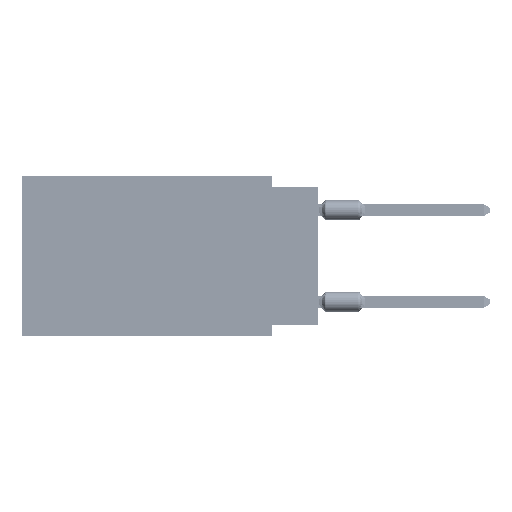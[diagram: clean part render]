
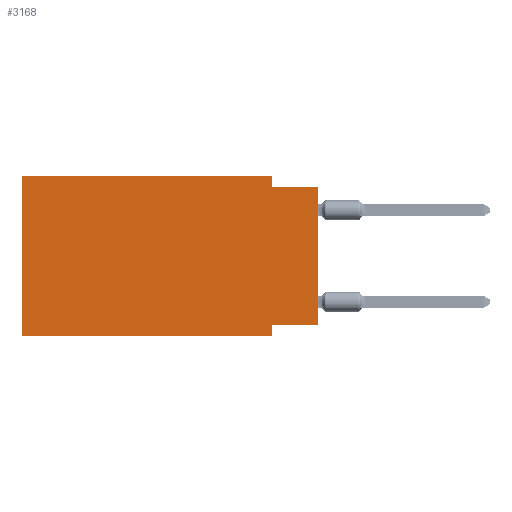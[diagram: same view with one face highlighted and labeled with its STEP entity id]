
A CAD part, left-side view. The second image highlights one B-rep face of the part: STEP entity #3168.
In plain terms, the highlighted planar face has unit normal (-1, 0, 0).
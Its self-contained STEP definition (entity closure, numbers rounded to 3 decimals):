
#1804 = VECTOR ( 'NONE', #104133, 1000. ) ;
#2034 = EDGE_CURVE ( 'NONE', #8779, #92417, #47428, .T. ) ;
#2912 = CARTESIAN_POINT ( 'NONE',  ( 0., 16.383, -8.89 ) ) ;
#3168 = ADVANCED_FACE ( 'NONE', ( #45358 ), #28938, .F. ) ;
#7784 = ORIENTED_EDGE ( 'NONE', *, *, #20127, .T. ) ;
#8779 = VERTEX_POINT ( 'NONE', #37899 ) ;
#11572 = ORIENTED_EDGE ( 'NONE', *, *, #51836, .F. ) ;
#13148 = ORIENTED_EDGE ( 'NONE', *, *, #77947, .F. ) ;
#14247 = DIRECTION ( 'NONE',  ( 0., -1., 0. ) ) ;
#14789 = VECTOR ( 'NONE', #48491, 1000. ) ;
#17339 = VERTEX_POINT ( 'NONE', #75725 ) ;
#20127 = EDGE_CURVE ( 'NONE', #87965, #74769, #34711, .T. ) ;
#21011 = DIRECTION ( 'NONE',  ( 1., 0., 0. ) ) ;
#26258 = EDGE_CURVE ( 'NONE', #67999, #33209, #50762, .T. ) ;
#26280 = CARTESIAN_POINT ( 'NONE',  ( 0., 16.383, -8.89 ) ) ;
#26295 = VECTOR ( 'NONE', #99499, 1000. ) ;
#27564 = CARTESIAN_POINT ( 'NONE',  ( 0., 2.54, -8.255 ) ) ;
#28281 = EDGE_CURVE ( 'NONE', #92417, #17339, #39917, .T. ) ;
#28938 = PLANE ( 'NONE',  #81557 ) ;
#29071 = CARTESIAN_POINT ( 'NONE',  ( 0., 16.383, 0. ) ) ;
#33209 = VERTEX_POINT ( 'NONE', #27564 ) ;
#34711 = LINE ( 'NONE', #2912, #74892 ) ;
#36169 = EDGE_LOOP ( 'NONE', ( #53392, #39734, #96352, #13148, #97157, #7784, #11572, #40665 ) ) ;
#37899 = CARTESIAN_POINT ( 'NONE',  ( 0., 2.54, 0. ) ) ;
#39734 = ORIENTED_EDGE ( 'NONE', *, *, #28281, .F. ) ;
#39737 = CARTESIAN_POINT ( 'NONE',  ( 0., 2.54, -0.635 ) ) ;
#39917 = LINE ( 'NONE', #71740, #100987 ) ;
#40665 = ORIENTED_EDGE ( 'NONE', *, *, #26258, .F. ) ;
#41595 = LINE ( 'NONE', #56988, #103772 ) ;
#45358 = FACE_OUTER_BOUND ( 'NONE', #36169, .T. ) ;
#47428 = LINE ( 'NONE', #82246, #1804 ) ;
#48491 = DIRECTION ( 'NONE',  ( 0., 0., 1. ) ) ;
#49646 = CARTESIAN_POINT ( 'NONE',  ( 0., 0., -8.255 ) ) ;
#50762 = LINE ( 'NONE', #83106, #26295 ) ;
#51836 = EDGE_CURVE ( 'NONE', #33209, #74769, #41595, .T. ) ;
#52178 = LINE ( 'NONE', #94553, #97591 ) ;
#53312 = DIRECTION ( 'NONE',  ( 0., 0., -1. ) ) ;
#53392 = ORIENTED_EDGE ( 'NONE', *, *, #82528, .T. ) ;
#54285 = DIRECTION ( 'NONE',  ( 0., 0., 1. ) ) ;
#56531 = EDGE_CURVE ( 'NONE', #87965, #81374, #64407, .T. ) ;
#56988 = CARTESIAN_POINT ( 'NONE',  ( 0., 2.54, -8.89 ) ) ;
#64407 = LINE ( 'NONE', #72886, #14789 ) ;
#67553 = DIRECTION ( 'NONE',  ( 0., -1., 0. ) ) ;
#67999 = VERTEX_POINT ( 'NONE', #49646 ) ;
#71740 = CARTESIAN_POINT ( 'NONE',  ( 0., 0., -0.635 ) ) ;
#72886 = CARTESIAN_POINT ( 'NONE',  ( 0., 16.383, 0. ) ) ;
#73831 = CARTESIAN_POINT ( 'NONE',  ( 0., 2.54, -8.89 ) ) ;
#74769 = VERTEX_POINT ( 'NONE', #73831 ) ;
#74892 = VECTOR ( 'NONE', #67553, 1000. ) ;
#75725 = CARTESIAN_POINT ( 'NONE',  ( 0., 0., -0.635 ) ) ;
#77947 = EDGE_CURVE ( 'NONE', #81374, #8779, #94767, .T. ) ;
#81374 = VERTEX_POINT ( 'NONE', #84478 ) ;
#81557 = AXIS2_PLACEMENT_3D ( 'NONE', #93572, #21011, #53312 ) ;
#82246 = CARTESIAN_POINT ( 'NONE',  ( 0., 2.54, 0. ) ) ;
#82528 = EDGE_CURVE ( 'NONE', #67999, #17339, #52178, .T. ) ;
#83106 = CARTESIAN_POINT ( 'NONE',  ( 0., 0., -8.255 ) ) ;
#84478 = CARTESIAN_POINT ( 'NONE',  ( 0., 16.383, 0. ) ) ;
#87965 = VERTEX_POINT ( 'NONE', #26280 ) ;
#89710 = DIRECTION ( 'NONE',  ( 0., -1., 0. ) ) ;
#92417 = VERTEX_POINT ( 'NONE', #39737 ) ;
#93572 = CARTESIAN_POINT ( 'NONE',  ( 0., 16.383, 0. ) ) ;
#94553 = CARTESIAN_POINT ( 'NONE',  ( 0., 0., 0. ) ) ;
#94767 = LINE ( 'NONE', #29071, #103810 ) ;
#96352 = ORIENTED_EDGE ( 'NONE', *, *, #2034, .F. ) ;
#97157 = ORIENTED_EDGE ( 'NONE', *, *, #56531, .F. ) ;
#97591 = VECTOR ( 'NONE', #54285, 1000. ) ;
#99499 = DIRECTION ( 'NONE',  ( 0., 1., 0. ) ) ;
#100987 = VECTOR ( 'NONE', #89710, 1000. ) ;
#103772 = VECTOR ( 'NONE', #104672, 1000. ) ;
#103810 = VECTOR ( 'NONE', #14247, 1000. ) ;
#104133 = DIRECTION ( 'NONE',  ( 0., 0., -1. ) ) ;
#104672 = DIRECTION ( 'NONE',  ( 0., 0., -1. ) ) ;
